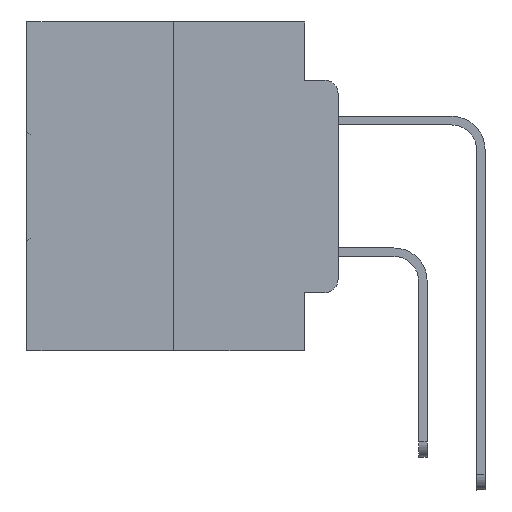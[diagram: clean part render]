
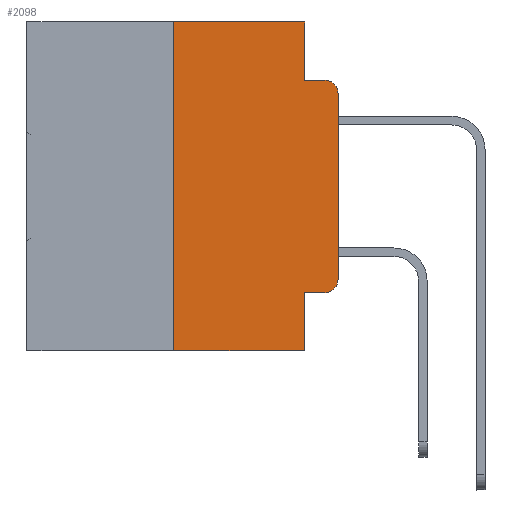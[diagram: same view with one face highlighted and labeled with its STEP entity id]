
A CAD part, left-side view. The second image highlights one B-rep face of the part: STEP entity #2098.
In plain terms, the highlighted planar face has unit normal (-1, 0, 0).
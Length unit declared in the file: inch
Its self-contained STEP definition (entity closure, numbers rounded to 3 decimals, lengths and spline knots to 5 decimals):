
#473 = AXIS2_PLACEMENT_3D ( 'NONE', #11307, #5507, #22342 ) ;
#537 = CARTESIAN_POINT ( 'NONE',  ( 0., 0.02, -0.3915 ) ) ;
#1172 = EDGE_LOOP ( 'NONE', ( #19722, #19366, #3191, #6478, #20582, #21011, #9430, #21438, #29815, #2505 ) ) ;
#1222 = VECTOR ( 'NONE', #33501, 39.37008 ) ;
#1910 = VERTEX_POINT ( 'NONE', #11578 ) ;
#1911 = CARTESIAN_POINT ( 'NONE',  ( 0., 0.051, -0.4115 ) ) ;
#2098 = ADVANCED_FACE ( 'NONE', ( #2447 ), #27580, .F. ) ;
#2447 = FACE_OUTER_BOUND ( 'NONE', #1172, .T. ) ;
#2505 = ORIENTED_EDGE ( 'NONE', *, *, #30389, .T. ) ;
#2545 = DIRECTION ( 'NONE',  ( 0., -1., 0. ) ) ;
#2993 = CARTESIAN_POINT ( 'NONE',  ( 0., 0.051, 0. ) ) ;
#3089 = EDGE_CURVE ( 'NONE', #12501, #1910, #5242, .T. ) ;
#3191 = ORIENTED_EDGE ( 'NONE', *, *, #11484, .F. ) ;
#3233 = DIRECTION ( 'NONE',  ( 0., 0., -1. ) ) ;
#3427 = AXIS2_PLACEMENT_3D ( 'NONE', #19959, #4156, #22520 ) ;
#3758 = EDGE_CURVE ( 'NONE', #32085, #19625, #4784, .T. ) ;
#4156 = DIRECTION ( 'NONE',  ( -1., 0., 0. ) ) ;
#4342 = CARTESIAN_POINT ( 'NONE',  ( 0., 0.02, -0.4115 ) ) ;
#4420 = DIRECTION ( 'NONE',  ( 0., 0., -1. ) ) ;
#4784 = LINE ( 'NONE', #24163, #24888 ) ;
#5242 = LINE ( 'NONE', #16973, #31295 ) ;
#5507 = DIRECTION ( 'NONE',  ( 1., 0., 0. ) ) ;
#5907 = EDGE_CURVE ( 'NONE', #19156, #1910, #13345, .T. ) ;
#6207 = CARTESIAN_POINT ( 'NONE',  ( 0., 0.25, 0. ) ) ;
#6248 = AXIS2_PLACEMENT_3D ( 'NONE', #537, #19087, #3233 ) ;
#6478 = ORIENTED_EDGE ( 'NONE', *, *, #3758, .F. ) ;
#7054 = DIRECTION ( 'NONE',  ( 0., 0., 1. ) ) ;
#7166 = CIRCLE ( 'NONE', #3427, 0.02 ) ;
#8027 = CARTESIAN_POINT ( 'NONE',  ( 0., 0., -0.3915 ) ) ;
#8567 = EDGE_CURVE ( 'NONE', #25430, #28717, #17995, .T. ) ;
#9384 = LINE ( 'NONE', #31728, #22556 ) ;
#9430 = ORIENTED_EDGE ( 'NONE', *, *, #5907, .T. ) ;
#10298 = CARTESIAN_POINT ( 'NONE',  ( 0., 0.25, -0.5 ) ) ;
#11255 = LINE ( 'NONE', #18920, #25176 ) ;
#11307 = CARTESIAN_POINT ( 'NONE',  ( 0., 0.473, 0. ) ) ;
#11484 = EDGE_CURVE ( 'NONE', #19625, #32461, #9384, .T. ) ;
#11578 = CARTESIAN_POINT ( 'NONE',  ( 0., 0.051, -0.5 ) ) ;
#11889 = CARTESIAN_POINT ( 'NONE',  ( 0., 0., -0.1085 ) ) ;
#12501 = VERTEX_POINT ( 'NONE', #1911 ) ;
#13345 = LINE ( 'NONE', #17418, #32313 ) ;
#14112 = VECTOR ( 'NONE', #2545, 39.37008 ) ;
#14769 = DIRECTION ( 'NONE',  ( 0., -1., 0. ) ) ;
#15037 = CARTESIAN_POINT ( 'NONE',  ( 0., 0.02, -0.0885 ) ) ;
#15756 = EDGE_CURVE ( 'NONE', #28717, #32461, #7166, .T. ) ;
#16973 = CARTESIAN_POINT ( 'NONE',  ( 0., 0.051, 0. ) ) ;
#17314 = CIRCLE ( 'NONE', #6248, 0.02 ) ;
#17418 = CARTESIAN_POINT ( 'NONE',  ( 0., 0.473, -0.5 ) ) ;
#17995 = LINE ( 'NONE', #22794, #18821 ) ;
#18013 = EDGE_CURVE ( 'NONE', #23324, #32085, #21060, .T. ) ;
#18821 = VECTOR ( 'NONE', #7054, 39.37008 ) ;
#18920 = CARTESIAN_POINT ( 'NONE',  ( 0., 0.051, -0.4115 ) ) ;
#19087 = DIRECTION ( 'NONE',  ( -1., 0., 0. ) ) ;
#19156 = VERTEX_POINT ( 'NONE', #10298 ) ;
#19366 = ORIENTED_EDGE ( 'NONE', *, *, #15756, .T. ) ;
#19625 = VERTEX_POINT ( 'NONE', #26489 ) ;
#19722 = ORIENTED_EDGE ( 'NONE', *, *, #8567, .T. ) ;
#19959 = CARTESIAN_POINT ( 'NONE',  ( 0., 0.02, -0.1085 ) ) ;
#20582 = ORIENTED_EDGE ( 'NONE', *, *, #18013, .F. ) ;
#21011 = ORIENTED_EDGE ( 'NONE', *, *, #28280, .F. ) ;
#21060 = LINE ( 'NONE', #31123, #14112 ) ;
#21438 = ORIENTED_EDGE ( 'NONE', *, *, #3089, .F. ) ;
#22342 = DIRECTION ( 'NONE',  ( 0., 0., -1. ) ) ;
#22491 = DIRECTION ( 'NONE',  ( 0., 0., -1. ) ) ;
#22520 = DIRECTION ( 'NONE',  ( 0., 0., -1. ) ) ;
#22556 = VECTOR ( 'NONE', #29281, 39.37008 ) ;
#22794 = CARTESIAN_POINT ( 'NONE',  ( 0., 0., 0. ) ) ;
#23324 = VERTEX_POINT ( 'NONE', #6207 ) ;
#24163 = CARTESIAN_POINT ( 'NONE',  ( 0., 0.051, 0. ) ) ;
#24888 = VECTOR ( 'NONE', #4420, 39.37008 ) ;
#25176 = VECTOR ( 'NONE', #29084, 39.37008 ) ;
#25430 = VERTEX_POINT ( 'NONE', #8027 ) ;
#26489 = CARTESIAN_POINT ( 'NONE',  ( 0., 0.051, -0.0885 ) ) ;
#27580 = PLANE ( 'NONE',  #473 ) ;
#28280 = EDGE_CURVE ( 'NONE', #19156, #23324, #30638, .T. ) ;
#28717 = VERTEX_POINT ( 'NONE', #11889 ) ;
#29084 = DIRECTION ( 'NONE',  ( 0., -1., 0. ) ) ;
#29281 = DIRECTION ( 'NONE',  ( 0., -1., 0. ) ) ;
#29815 = ORIENTED_EDGE ( 'NONE', *, *, #32763, .T. ) ;
#30389 = EDGE_CURVE ( 'NONE', #32429, #25430, #17314, .T. ) ;
#30638 = LINE ( 'NONE', #30925, #1222 ) ;
#30925 = CARTESIAN_POINT ( 'NONE',  ( 0., 0.25, 0. ) ) ;
#31123 = CARTESIAN_POINT ( 'NONE',  ( 0., 0.473, 0. ) ) ;
#31295 = VECTOR ( 'NONE', #22491, 39.37008 ) ;
#31728 = CARTESIAN_POINT ( 'NONE',  ( 0., 0.051, -0.0885 ) ) ;
#32085 = VERTEX_POINT ( 'NONE', #2993 ) ;
#32313 = VECTOR ( 'NONE', #14769, 39.37008 ) ;
#32429 = VERTEX_POINT ( 'NONE', #4342 ) ;
#32461 = VERTEX_POINT ( 'NONE', #15037 ) ;
#32763 = EDGE_CURVE ( 'NONE', #12501, #32429, #11255, .T. ) ;
#33501 = DIRECTION ( 'NONE',  ( 0., 0., 1. ) ) ;
